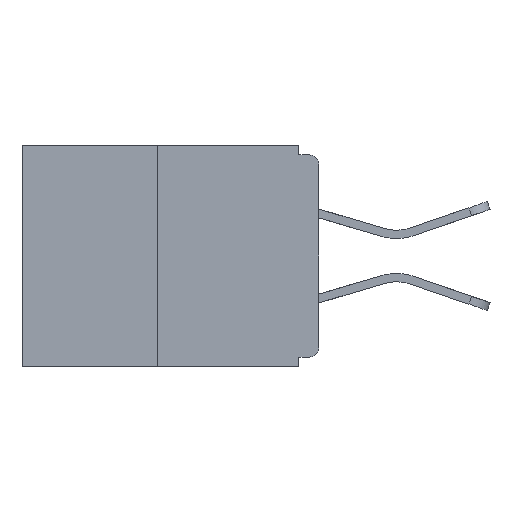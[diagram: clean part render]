
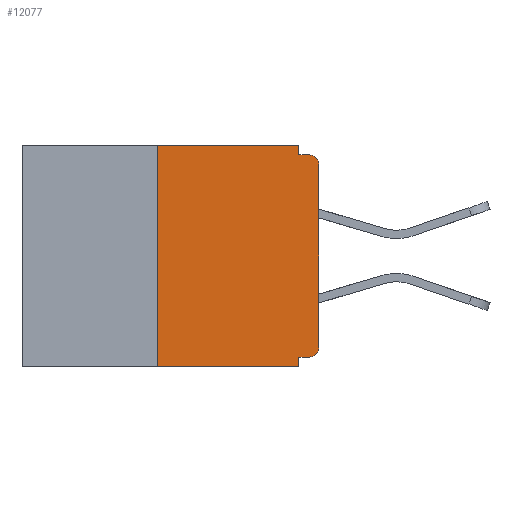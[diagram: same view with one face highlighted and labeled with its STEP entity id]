
A CAD part, left-side view. The second image highlights one B-rep face of the part: STEP entity #12077.
In plain terms, the highlighted planar face has unit normal (-1, 0, 0).
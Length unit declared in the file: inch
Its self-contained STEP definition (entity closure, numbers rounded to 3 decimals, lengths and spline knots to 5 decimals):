
#674 = CARTESIAN_POINT ( 'NONE',  ( 0., 0.25, -0.343 ) ) ;
#711 = DIRECTION ( 'NONE',  ( 0., 0., -1. ) ) ;
#1530 = CARTESIAN_POINT ( 'NONE',  ( 0., 0.46, 0. ) ) ;
#1802 = CARTESIAN_POINT ( 'NONE',  ( 0., 0., -0.313 ) ) ;
#1818 = VERTEX_POINT ( 'NONE', #1802 ) ;
#2114 = PLANE ( 'NONE',  #7485 ) ;
#2637 = ORIENTED_EDGE ( 'NONE', *, *, #2758, .F. ) ;
#2697 = FACE_OUTER_BOUND ( 'NONE', #4576, .T. ) ;
#2713 = EDGE_CURVE ( 'NONE', #17805, #6769, #11020, .T. ) ;
#2758 = EDGE_CURVE ( 'NONE', #6939, #16997, #14064, .T. ) ;
#2934 = CARTESIAN_POINT ( 'NONE',  ( 0., 0., -0.328 ) ) ;
#3251 = DIRECTION ( 'NONE',  ( -1., 0., 0. ) ) ;
#3497 = LINE ( 'NONE', #6016, #7009 ) ;
#3802 = DIRECTION ( 'NONE',  ( 0., -1., 0. ) ) ;
#3939 = ORIENTED_EDGE ( 'NONE', *, *, #2713, .F. ) ;
#4022 = ORIENTED_EDGE ( 'NONE', *, *, #10193, .F. ) ;
#4088 = CIRCLE ( 'NONE', #7418, 0.015 ) ;
#4153 = ORIENTED_EDGE ( 'NONE', *, *, #16239, .F. ) ;
#4281 = CARTESIAN_POINT ( 'NONE',  ( 0., 0.031, 0. ) ) ;
#4576 = EDGE_LOOP ( 'NONE', ( #3939, #4022, #13081, #2637, #4153, #5706, #16698, #18811, #6187, #11353 ) ) ;
#4579 = VECTOR ( 'NONE', #3802, 39.37008 ) ;
#4817 = LINE ( 'NONE', #15885, #4579 ) ;
#4931 = AXIS2_PLACEMENT_3D ( 'NONE', #12442, #3251, #12322 ) ;
#5249 = DIRECTION ( 'NONE',  ( 0., 0., -1. ) ) ;
#5706 = ORIENTED_EDGE ( 'NONE', *, *, #7589, .T. ) ;
#5826 = CARTESIAN_POINT ( 'NONE',  ( 0., 0.031, -0.343 ) ) ;
#5905 = DIRECTION ( 'NONE',  ( 1., 0., 0. ) ) ;
#6016 = CARTESIAN_POINT ( 'NONE',  ( 0., 0.25, 0. ) ) ;
#6044 = EDGE_CURVE ( 'NONE', #1818, #9098, #8857, .T. ) ;
#6187 = ORIENTED_EDGE ( 'NONE', *, *, #6476, .F. ) ;
#6476 = EDGE_CURVE ( 'NONE', #17267, #6657, #15217, .T. ) ;
#6502 = DIRECTION ( 'NONE',  ( 0., -1., 0. ) ) ;
#6657 = VERTEX_POINT ( 'NONE', #8549 ) ;
#6769 = VERTEX_POINT ( 'NONE', #4281 ) ;
#6939 = VERTEX_POINT ( 'NONE', #16170 ) ;
#7009 = VECTOR ( 'NONE', #8993, 39.37008 ) ;
#7418 = AXIS2_PLACEMENT_3D ( 'NONE', #18790, #14243, #5249 ) ;
#7485 = AXIS2_PLACEMENT_3D ( 'NONE', #1530, #5905, #10456 ) ;
#7589 = EDGE_CURVE ( 'NONE', #10603, #1818, #4088, .T. ) ;
#7612 = EDGE_CURVE ( 'NONE', #15973, #16997, #4817, .T. ) ;
#8549 = CARTESIAN_POINT ( 'NONE',  ( 0., 0.015, -0.015 ) ) ;
#8857 = LINE ( 'NONE', #18883, #19511 ) ;
#8887 = LINE ( 'NONE', #2934, #18370 ) ;
#8993 = DIRECTION ( 'NONE',  ( 0., 0., 1. ) ) ;
#9098 = VERTEX_POINT ( 'NONE', #11751 ) ;
#9381 = VECTOR ( 'NONE', #17922, 39.37008 ) ;
#9607 = VECTOR ( 'NONE', #15036, 39.37008 ) ;
#10193 = EDGE_CURVE ( 'NONE', #15973, #17805, #3497, .T. ) ;
#10456 = DIRECTION ( 'NONE',  ( 0., 0., -1. ) ) ;
#10603 = VERTEX_POINT ( 'NONE', #18078 ) ;
#11020 = LINE ( 'NONE', #17503, #9381 ) ;
#11057 = CARTESIAN_POINT ( 'NONE',  ( 0., 0., -0.015 ) ) ;
#11353 = ORIENTED_EDGE ( 'NONE', *, *, #14087, .F. ) ;
#11553 = LINE ( 'NONE', #15681, #18222 ) ;
#11751 = CARTESIAN_POINT ( 'NONE',  ( 0., 0., -0.03 ) ) ;
#12008 = DIRECTION ( 'NONE',  ( 0., 1., 0. ) ) ;
#12077 = ADVANCED_FACE ( 'NONE', ( #2697 ), #2114, .F. ) ;
#12322 = DIRECTION ( 'NONE',  ( 0., 0., -1. ) ) ;
#12442 = CARTESIAN_POINT ( 'NONE',  ( 0., 0.015, -0.03 ) ) ;
#12852 = CIRCLE ( 'NONE', #4931, 0.015 ) ;
#13081 = ORIENTED_EDGE ( 'NONE', *, *, #7612, .T. ) ;
#14064 = LINE ( 'NONE', #5826, #9607 ) ;
#14087 = EDGE_CURVE ( 'NONE', #6769, #17267, #11553, .T. ) ;
#14243 = DIRECTION ( 'NONE',  ( -1., 0., 0. ) ) ;
#14524 = CARTESIAN_POINT ( 'NONE',  ( 0., 0.031, -0.343 ) ) ;
#15036 = DIRECTION ( 'NONE',  ( 0., 0., -1. ) ) ;
#15217 = LINE ( 'NONE', #11057, #15427 ) ;
#15427 = VECTOR ( 'NONE', #6502, 39.37008 ) ;
#15681 = CARTESIAN_POINT ( 'NONE',  ( 0., 0.031, 0. ) ) ;
#15885 = CARTESIAN_POINT ( 'NONE',  ( 0., 0.46, -0.343 ) ) ;
#15973 = VERTEX_POINT ( 'NONE', #674 ) ;
#16170 = CARTESIAN_POINT ( 'NONE',  ( 0., 0.031, -0.328 ) ) ;
#16239 = EDGE_CURVE ( 'NONE', #10603, #6939, #8887, .T. ) ;
#16260 = CARTESIAN_POINT ( 'NONE',  ( 0., 0.25, 0. ) ) ;
#16698 = ORIENTED_EDGE ( 'NONE', *, *, #6044, .T. ) ;
#16997 = VERTEX_POINT ( 'NONE', #14524 ) ;
#17267 = VERTEX_POINT ( 'NONE', #17289 ) ;
#17289 = CARTESIAN_POINT ( 'NONE',  ( 0., 0.031, -0.015 ) ) ;
#17461 = DIRECTION ( 'NONE',  ( 0., 0., 1. ) ) ;
#17466 = EDGE_CURVE ( 'NONE', #9098, #6657, #12852, .T. ) ;
#17503 = CARTESIAN_POINT ( 'NONE',  ( 0., 0.46, 0. ) ) ;
#17805 = VERTEX_POINT ( 'NONE', #16260 ) ;
#17922 = DIRECTION ( 'NONE',  ( 0., -1., 0. ) ) ;
#18078 = CARTESIAN_POINT ( 'NONE',  ( 0., 0.015, -0.328 ) ) ;
#18222 = VECTOR ( 'NONE', #711, 39.37008 ) ;
#18370 = VECTOR ( 'NONE', #12008, 39.37008 ) ;
#18790 = CARTESIAN_POINT ( 'NONE',  ( 0., 0.015, -0.313 ) ) ;
#18811 = ORIENTED_EDGE ( 'NONE', *, *, #17466, .T. ) ;
#18883 = CARTESIAN_POINT ( 'NONE',  ( 0., 0., 0. ) ) ;
#19511 = VECTOR ( 'NONE', #17461, 39.37008 ) ;
